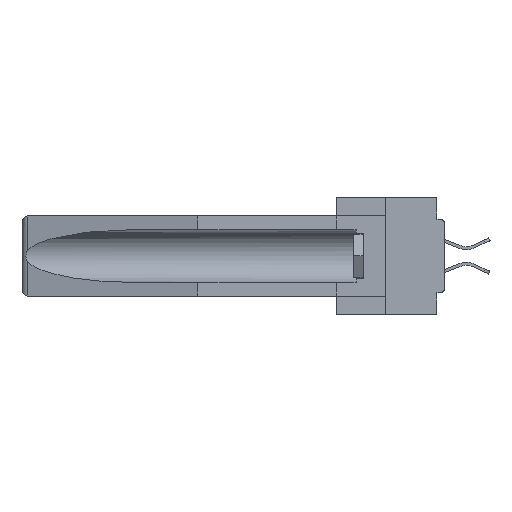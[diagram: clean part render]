
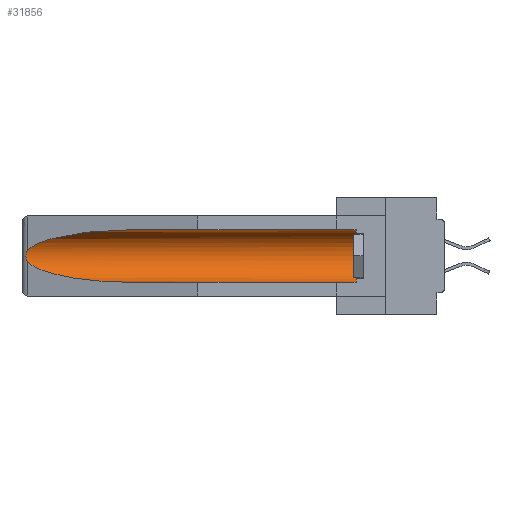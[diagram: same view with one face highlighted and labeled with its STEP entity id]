
A CAD part, left-side view. The second image highlights one B-rep face of the part: STEP entity #31856.
In plain terms, the highlighted cylindrical face has radius 2.857 mm (diameter 5.715 mm), a partial arc.
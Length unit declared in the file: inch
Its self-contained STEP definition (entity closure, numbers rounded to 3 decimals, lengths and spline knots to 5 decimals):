
#361 = EDGE_CURVE ( 'NONE', #29686, #32938, #441, .T. ) ;
#441 = LINE ( 'NONE', #34221, #11407 ) ;
#811 = AXIS2_PLACEMENT_3D ( 'NONE', #13905, #29244, #20006 ) ;
#2431 = CARTESIAN_POINT ( 'NONE',  ( 0.26597, 1.52961, -0.15275 ) ) ;
#4156 = ORIENTED_EDGE ( 'NONE', *, *, #361, .F. ) ;
#4232 = ORIENTED_EDGE ( 'NONE', *, *, #9009, .T. ) ;
#4770 = CYLINDRICAL_SURFACE ( 'NONE', #811, 0.1125 ) ;
#5058 = CARTESIAN_POINT ( 'NONE',  ( 0.25451, 1.48313, -0.09465 ) ) ;
#6438 = EDGE_CURVE ( 'NONE', #14560, #36452, #15389, .T. ) ;
#6510 = DIRECTION ( 'NONE',  ( 0., 1., 0. ) ) ;
#6987 = CARTESIAN_POINT ( 'NONE',  ( 0.26537, 1.52718, -0.14972 ) ) ;
#7063 = CARTESIAN_POINT ( 'NONE',  ( 0.155, -0.30754, -0.059 ) ) ;
#8170 = DIRECTION ( 'NONE',  ( 0., 0., 1. ) ) ;
#8511 = CARTESIAN_POINT ( 'NONE',  ( 0.26537, 1.52718, -0.19328 ) ) ;
#9009 = EDGE_CURVE ( 'NONE', #29686, #34867, #36324, .T. ) ;
#9957 = EDGE_LOOP ( 'NONE', ( #35171, #37465, #22213, #4156, #4232, #20099 ) ) ;
#11407 = VECTOR ( 'NONE', #6510, 39.37008 ) ;
#11611 = CARTESIAN_POINT ( 'NONE',  ( 0.26537, 1.52718, -0.14972 ) ) ;
#13192 =( BOUNDED_CURVE ( )  B_SPLINE_CURVE ( 3, ( #14018, #35447, #17178, #22929 ),
 .UNSPECIFIED., .F., .F. ) 
 B_SPLINE_CURVE_WITH_KNOTS ( ( 4, 4 ),
 ( 0.1948, 1.5708 ),
 .UNSPECIFIED. ) 
 CURVE ( )  GEOMETRIC_REPRESENTATION_ITEM ( )  RATIONAL_B_SPLINE_CURVE ( ( 1., 0.848, 0.848, 1. ) ) 
 REPRESENTATION_ITEM ( '' )  );
#13905 = CARTESIAN_POINT ( 'NONE',  ( 0.155, -0.30754, -0.1715 ) ) ;
#14018 = CARTESIAN_POINT ( 'NONE',  ( 0.26537, 1.52718, -0.19328 ) ) ;
#14046 = CARTESIAN_POINT ( 'NONE',  ( 0.2675, 1.53308, -0.16763 ) ) ;
#14560 = VERTEX_POINT ( 'NONE', #26676 ) ;
#15389 =( BOUNDED_CURVE ( )  B_SPLINE_CURVE ( 3, ( #23447, #35309, #5058, #17322 ),
 .UNSPECIFIED., .F., .F. ) 
 B_SPLINE_CURVE_WITH_KNOTS ( ( 4, 4 ),
 ( 4.71239, 6.08839 ),
 .UNSPECIFIED. ) 
 CURVE ( )  GEOMETRIC_REPRESENTATION_ITEM ( )  RATIONAL_B_SPLINE_CURVE ( ( 1., 0.848, 0.848, 1. ) ) 
 REPRESENTATION_ITEM ( '' )  );
#17178 = CARTESIAN_POINT ( 'NONE',  ( 0.21114, 1.30732, -0.284 ) ) ;
#17322 = CARTESIAN_POINT ( 'NONE',  ( 0.26537, 1.52718, -0.14972 ) ) ;
#17337 = B_SPLINE_CURVE_WITH_KNOTS ( 'NONE', 3,
 ( #11611, #2431, #26556, #35862, #14046, #26284, #20405, #38497, #35730, #29368 ),
 .UNSPECIFIED., .F., .F.,
 ( 4, 2, 2, 2, 4 ),
 ( 0., 0.00029, 0.00058, 0.00087, 0.00117 ),
 .UNSPECIFIED. ) ;
#19425 = DIRECTION ( 'NONE',  ( 0., 1., 0. ) ) ;
#20006 = DIRECTION ( 'NONE',  ( 0., 0., 1. ) ) ;
#20099 = ORIENTED_EDGE ( 'NONE', *, *, #31210, .T. ) ;
#20405 = CARTESIAN_POINT ( 'NONE',  ( 0.2673, 1.53269, -0.17917 ) ) ;
#22213 = ORIENTED_EDGE ( 'NONE', *, *, #24387, .T. ) ;
#22929 = CARTESIAN_POINT ( 'NONE',  ( 0.155, 1.07973, -0.284 ) ) ;
#23144 = CARTESIAN_POINT ( 'NONE',  ( 0.155, 0.126, -0.284 ) ) ;
#23357 = CARTESIAN_POINT ( 'NONE',  ( 0.155, 0.126, -0.1715 ) ) ;
#23447 = CARTESIAN_POINT ( 'NONE',  ( 0.155, 1.07973, -0.059 ) ) ;
#23827 = FACE_OUTER_BOUND ( 'NONE', #9957, .T. ) ;
#24061 = VECTOR ( 'NONE', #19425, 39.37008 ) ;
#24387 = EDGE_CURVE ( 'NONE', #26054, #32938, #13192, .T. ) ;
#24563 = CARTESIAN_POINT ( 'NONE',  ( 0.155, 0.126, -0.059 ) ) ;
#25558 = AXIS2_PLACEMENT_3D ( 'NONE', #23357, #38801, #8170 ) ;
#25609 = EDGE_CURVE ( 'NONE', #36452, #26054, #17337, .T. ) ;
#26054 = VERTEX_POINT ( 'NONE', #8511 ) ;
#26284 = CARTESIAN_POINT ( 'NONE',  ( 0.2675, 1.53308, -0.17534 ) ) ;
#26556 = CARTESIAN_POINT ( 'NONE',  ( 0.26654, 1.53092, -0.15636 ) ) ;
#26676 = CARTESIAN_POINT ( 'NONE',  ( 0.155, 1.07973, -0.059 ) ) ;
#29244 = DIRECTION ( 'NONE',  ( 0., 1., 0. ) ) ;
#29368 = CARTESIAN_POINT ( 'NONE',  ( 0.26537, 1.52718, -0.19328 ) ) ;
#29686 = VERTEX_POINT ( 'NONE', #23144 ) ;
#31210 = EDGE_CURVE ( 'NONE', #34867, #14560, #37881, .T. ) ;
#31856 = ADVANCED_FACE ( 'NONE', ( #23827 ), #4770, .F. ) ;
#32938 = VERTEX_POINT ( 'NONE', #34102 ) ;
#34102 = CARTESIAN_POINT ( 'NONE',  ( 0.155, 1.07973, -0.284 ) ) ;
#34221 = CARTESIAN_POINT ( 'NONE',  ( 0.155, -0.30754, -0.284 ) ) ;
#34867 = VERTEX_POINT ( 'NONE', #24563 ) ;
#35171 = ORIENTED_EDGE ( 'NONE', *, *, #6438, .T. ) ;
#35309 = CARTESIAN_POINT ( 'NONE',  ( 0.21114, 1.30732, -0.059 ) ) ;
#35447 = CARTESIAN_POINT ( 'NONE',  ( 0.25451, 1.48313, -0.24835 ) ) ;
#35730 = CARTESIAN_POINT ( 'NONE',  ( 0.26597, 1.5296, -0.19026 ) ) ;
#35862 = CARTESIAN_POINT ( 'NONE',  ( 0.2673, 1.5327, -0.16383 ) ) ;
#36324 = CIRCLE ( 'NONE', #25558, 0.1125 ) ;
#36452 = VERTEX_POINT ( 'NONE', #6987 ) ;
#37465 = ORIENTED_EDGE ( 'NONE', *, *, #25609, .T. ) ;
#37881 = LINE ( 'NONE', #7063, #24061 ) ;
#38497 = CARTESIAN_POINT ( 'NONE',  ( 0.26655, 1.53094, -0.18657 ) ) ;
#38801 = DIRECTION ( 'NONE',  ( 0., -1., 0. ) ) ;
